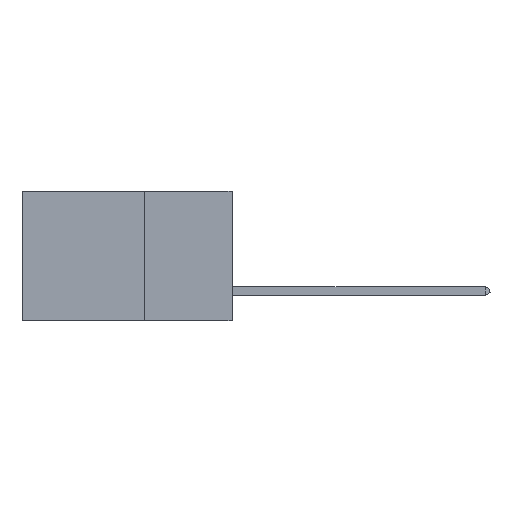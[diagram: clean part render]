
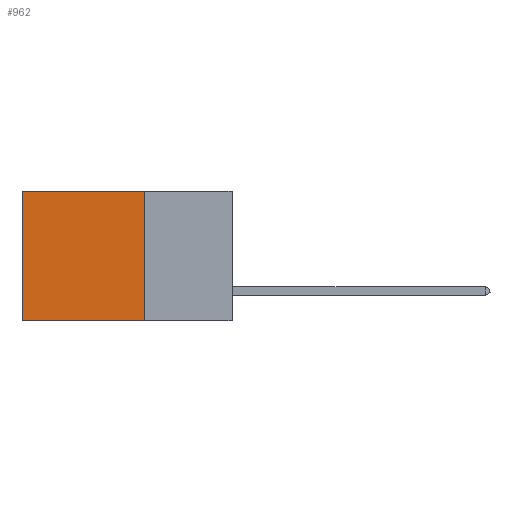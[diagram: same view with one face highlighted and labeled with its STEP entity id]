
A CAD part, left-side view. The second image highlights one B-rep face of the part: STEP entity #962.
In plain terms, the highlighted planar face has unit normal (-1, 0, 0).
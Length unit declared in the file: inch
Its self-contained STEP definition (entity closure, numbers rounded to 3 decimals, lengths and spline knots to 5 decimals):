
#298 = VERTEX_POINT ( 'NONE', #7430 ) ;
#745 = EDGE_CURVE ( 'NONE', #34731, #20897, #41581, .T. ) ;
#962 = ADVANCED_FACE ( 'NONE', ( #19690 ), #24432, .F. ) ;
#2046 = VERTEX_POINT ( 'NONE', #9696 ) ;
#2450 = DIRECTION ( 'NONE',  ( 0., 0., -1. ) ) ;
#4894 = ORIENTED_EDGE ( 'NONE', *, *, #19685, .T. ) ;
#6074 = EDGE_CURVE ( 'NONE', #298, #2046, #22736, .T. ) ;
#7171 = DIRECTION ( 'NONE',  ( 0., 1., 0. ) ) ;
#7430 = CARTESIAN_POINT ( 'NONE',  ( 0.2875, 0.25, 0. ) ) ;
#9696 = CARTESIAN_POINT ( 'NONE',  ( 0.2875, 0.6, 0. ) ) ;
#9884 = DIRECTION ( 'NONE',  ( 1., 0., 0. ) ) ;
#11643 = EDGE_CURVE ( 'NONE', #298, #34731, #34432, .T. ) ;
#12936 = CARTESIAN_POINT ( 'NONE',  ( 0.2875, 0.25, 0. ) ) ;
#15131 = VECTOR ( 'NONE', #7171, 39.37008 ) ;
#15837 = ORIENTED_EDGE ( 'NONE', *, *, #745, .F. ) ;
#16258 = CARTESIAN_POINT ( 'NONE',  ( 0.2875, 0.25, 0. ) ) ;
#17134 = EDGE_LOOP ( 'NONE', ( #4894, #15837, #41460, #32767 ) ) ;
#18418 = CARTESIAN_POINT ( 'NONE',  ( 0.2875, 0.25, 0. ) ) ;
#19685 = EDGE_CURVE ( 'NONE', #2046, #20897, #32444, .T. ) ;
#19690 = FACE_OUTER_BOUND ( 'NONE', #17134, .T. ) ;
#19814 = VECTOR ( 'NONE', #44770, 39.37008 ) ;
#20897 = VERTEX_POINT ( 'NONE', #36810 ) ;
#22736 = LINE ( 'NONE', #18418, #26183 ) ;
#23345 = AXIS2_PLACEMENT_3D ( 'NONE', #12936, #9884, #2450 ) ;
#24432 = PLANE ( 'NONE',  #23345 ) ;
#26095 = DIRECTION ( 'NONE',  ( 0., 1., 0. ) ) ;
#26183 = VECTOR ( 'NONE', #26095, 39.37008 ) ;
#28732 = CARTESIAN_POINT ( 'NONE',  ( 0.2875, 0.25, -0.37 ) ) ;
#29165 = CARTESIAN_POINT ( 'NONE',  ( 0.2875, 0.25, -0.37 ) ) ;
#32444 = LINE ( 'NONE', #36928, #19814 ) ;
#32767 = ORIENTED_EDGE ( 'NONE', *, *, #6074, .T. ) ;
#34432 = LINE ( 'NONE', #16258, #39604 ) ;
#34731 = VERTEX_POINT ( 'NONE', #28732 ) ;
#36810 = CARTESIAN_POINT ( 'NONE',  ( 0.2875, 0.6, -0.37 ) ) ;
#36928 = CARTESIAN_POINT ( 'NONE',  ( 0.2875, 0.6, 0. ) ) ;
#39604 = VECTOR ( 'NONE', #42105, 39.37008 ) ;
#41460 = ORIENTED_EDGE ( 'NONE', *, *, #11643, .F. ) ;
#41581 = LINE ( 'NONE', #29165, #15131 ) ;
#42105 = DIRECTION ( 'NONE',  ( 0., 0., -1. ) ) ;
#44770 = DIRECTION ( 'NONE',  ( 0., 0., -1. ) ) ;
